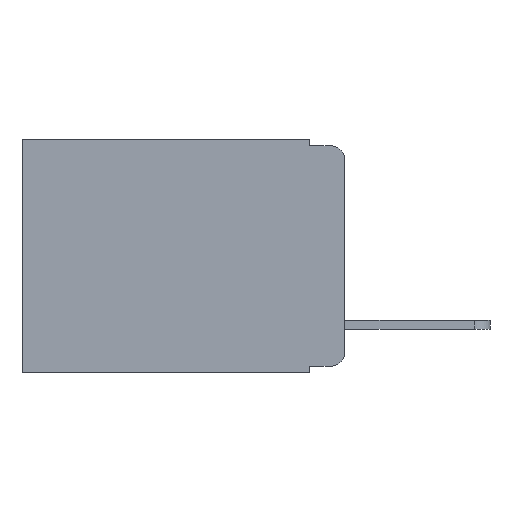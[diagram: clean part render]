
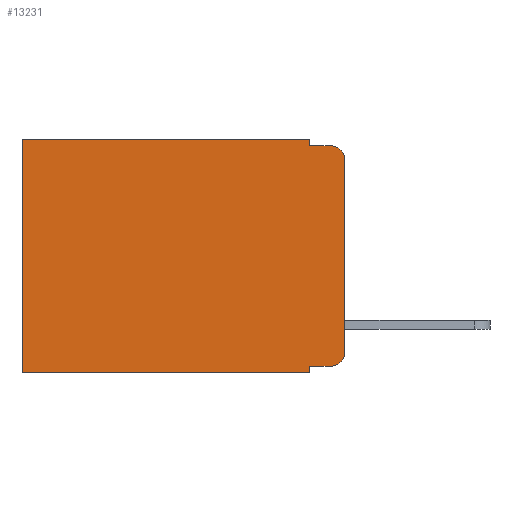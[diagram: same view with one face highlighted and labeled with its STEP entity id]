
A CAD part, left-side view. The second image highlights one B-rep face of the part: STEP entity #13231.
In plain terms, the highlighted planar face has unit normal (-1, 0, 0).
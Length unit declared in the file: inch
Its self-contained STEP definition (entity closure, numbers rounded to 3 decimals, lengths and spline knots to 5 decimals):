
#166 = VERTEX_POINT ( 'NONE', #2242 ) ;
#414 = DIRECTION ( 'NONE',  ( -1., 0., 0. ) ) ;
#461 = CARTESIAN_POINT ( 'NONE',  ( 0.298, 0.02, -0.313 ) ) ;
#696 = EDGE_CURVE ( 'NONE', #166, #11886, #8518, .T. ) ;
#703 = AXIS2_PLACEMENT_3D ( 'NONE', #461, #414, #753 ) ;
#723 = EDGE_CURVE ( 'NONE', #2849, #11886, #8712, .T. ) ;
#753 = DIRECTION ( 'NONE',  ( 0., 0., -1. ) ) ;
#799 = VERTEX_POINT ( 'NONE', #15249 ) ;
#801 = EDGE_CURVE ( 'NONE', #12892, #2849, #8092, .T. ) ;
#815 = LINE ( 'NONE', #8759, #3101 ) ;
#833 = EDGE_CURVE ( 'NONE', #5508, #7349, #8027, .T. ) ;
#957 = EDGE_CURVE ( 'NONE', #8709, #799, #6829, .T. ) ;
#1048 = DIRECTION ( 'NONE',  ( 0., 0., -1. ) ) ;
#1089 = LINE ( 'NONE', #3048, #8376 ) ;
#1217 = EDGE_CURVE ( 'NONE', #8709, #13309, #5358, .T. ) ;
#1345 = DIRECTION ( 'NONE',  ( 0., 0., -1. ) ) ;
#1729 = CIRCLE ( 'NONE', #703, 0.02 ) ;
#1810 = ORIENTED_EDGE ( 'NONE', *, *, #13506, .F. ) ;
#1923 = EDGE_CURVE ( 'NONE', #13309, #12483, #1729, .T. ) ;
#1992 = EDGE_CURVE ( 'NONE', #12892, #5508, #815, .T. ) ;
#2231 = ORIENTED_EDGE ( 'NONE', *, *, #696, .T. ) ;
#2242 = CARTESIAN_POINT ( 'NONE',  ( 0.298, 0., -0.03 ) ) ;
#2402 = ORIENTED_EDGE ( 'NONE', *, *, #723, .F. ) ;
#2849 = VERTEX_POINT ( 'NONE', #8165 ) ;
#2913 = ORIENTED_EDGE ( 'NONE', *, *, #801, .F. ) ;
#2930 = ORIENTED_EDGE ( 'NONE', *, *, #1992, .T. ) ;
#2931 = CARTESIAN_POINT ( 'NONE',  ( 0.298, 0.051, -0.333 ) ) ;
#2993 = DIRECTION ( 'NONE',  ( 0., 0., -1. ) ) ;
#3048 = CARTESIAN_POINT ( 'NONE',  ( 0.298, 0., 0. ) ) ;
#3101 = VECTOR ( 'NONE', #10884, 39.37008 ) ;
#3263 = DIRECTION ( 'NONE',  ( 0., -1., 0. ) ) ;
#3344 = ORIENTED_EDGE ( 'NONE', *, *, #833, .T. ) ;
#3425 = DIRECTION ( 'NONE',  ( 0., 0., -1. ) ) ;
#3850 = AXIS2_PLACEMENT_3D ( 'NONE', #15943, #15954, #3425 ) ;
#4925 = ORIENTED_EDGE ( 'NONE', *, *, #8509, .F. ) ;
#5118 = CARTESIAN_POINT ( 'NONE',  ( 0.298, 0.473, -0.343 ) ) ;
#5130 = ORIENTED_EDGE ( 'NONE', *, *, #957, .F. ) ;
#5151 = VECTOR ( 'NONE', #14199, 39.37008 ) ;
#5358 = LINE ( 'NONE', #2931, #5151 ) ;
#5508 = VERTEX_POINT ( 'NONE', #7726 ) ;
#5586 = DIRECTION ( 'NONE',  ( 0., 0., -1. ) ) ;
#5740 = ORIENTED_EDGE ( 'NONE', *, *, #1217, .T. ) ;
#6065 = CARTESIAN_POINT ( 'NONE',  ( 0.298, 0.02, -0.333 ) ) ;
#6096 = ORIENTED_EDGE ( 'NONE', *, *, #1923, .T. ) ;
#6161 = CARTESIAN_POINT ( 'NONE',  ( 0.298, 0., -0.343 ) ) ;
#6829 = LINE ( 'NONE', #15810, #6974 ) ;
#6974 = VECTOR ( 'NONE', #5586, 39.37008 ) ;
#7032 = DIRECTION ( 'NONE',  ( 0., 1., 0. ) ) ;
#7075 = LINE ( 'NONE', #6161, #16628 ) ;
#7100 = DIRECTION ( 'NONE',  ( 0., 0., -1. ) ) ;
#7160 = DIRECTION ( 'NONE',  ( 1., 0., 0. ) ) ;
#7166 = CARTESIAN_POINT ( 'NONE',  ( 0.298, 0., 0. ) ) ;
#7321 = PLANE ( 'NONE',  #7689 ) ;
#7349 = VERTEX_POINT ( 'NONE', #5118 ) ;
#7689 = AXIS2_PLACEMENT_3D ( 'NONE', #7166, #7160, #7100 ) ;
#7718 = VECTOR ( 'NONE', #1345, 39.37008 ) ;
#7726 = CARTESIAN_POINT ( 'NONE',  ( 0.298, 0.473, 0. ) ) ;
#8027 = LINE ( 'NONE', #16609, #7718 ) ;
#8043 = VECTOR ( 'NONE', #1048, 39.37008 ) ;
#8092 = LINE ( 'NONE', #16226, #8043 ) ;
#8165 = CARTESIAN_POINT ( 'NONE',  ( 0.298, 0.051, -0.01 ) ) ;
#8376 = VECTOR ( 'NONE', #2993, 39.37008 ) ;
#8384 = VECTOR ( 'NONE', #3263, 39.37008 ) ;
#8484 = CARTESIAN_POINT ( 'NONE',  ( 0.298, 0.051, -0.333 ) ) ;
#8509 = EDGE_CURVE ( 'NONE', #799, #7349, #7075, .T. ) ;
#8518 = CIRCLE ( 'NONE', #3850, 0.02 ) ;
#8709 = VERTEX_POINT ( 'NONE', #8484 ) ;
#8712 = LINE ( 'NONE', #16000, #8384 ) ;
#8759 = CARTESIAN_POINT ( 'NONE',  ( 0.298, 0., 0. ) ) ;
#9399 = EDGE_LOOP ( 'NONE', ( #1810, #2231, #2402, #2913, #2930, #3344, #4925, #5130, #5740, #6096 ) ) ;
#10169 = FACE_OUTER_BOUND ( 'NONE', #9399, .T. ) ;
#10884 = DIRECTION ( 'NONE',  ( 0., 1., 0. ) ) ;
#11520 = CARTESIAN_POINT ( 'NONE',  ( 0.298, 0.051, 0. ) ) ;
#11886 = VERTEX_POINT ( 'NONE', #14066 ) ;
#12483 = VERTEX_POINT ( 'NONE', #15736 ) ;
#12892 = VERTEX_POINT ( 'NONE', #11520 ) ;
#13231 = ADVANCED_FACE ( 'NONE', ( #10169 ), #7321, .F. ) ;
#13309 = VERTEX_POINT ( 'NONE', #6065 ) ;
#13506 = EDGE_CURVE ( 'NONE', #166, #12483, #1089, .T. ) ;
#14066 = CARTESIAN_POINT ( 'NONE',  ( 0.298, 0.02, -0.01 ) ) ;
#14199 = DIRECTION ( 'NONE',  ( 0., -1., 0. ) ) ;
#15249 = CARTESIAN_POINT ( 'NONE',  ( 0.298, 0.051, -0.343 ) ) ;
#15736 = CARTESIAN_POINT ( 'NONE',  ( 0.298, 0., -0.313 ) ) ;
#15810 = CARTESIAN_POINT ( 'NONE',  ( 0.298, 0.051, 0. ) ) ;
#15943 = CARTESIAN_POINT ( 'NONE',  ( 0.298, 0.02, -0.03 ) ) ;
#15954 = DIRECTION ( 'NONE',  ( -1., 0., 0. ) ) ;
#16000 = CARTESIAN_POINT ( 'NONE',  ( 0.298, 0.051, -0.01 ) ) ;
#16226 = CARTESIAN_POINT ( 'NONE',  ( 0.298, 0.051, 0. ) ) ;
#16609 = CARTESIAN_POINT ( 'NONE',  ( 0.298, 0.473, 0. ) ) ;
#16628 = VECTOR ( 'NONE', #7032, 39.37008 ) ;
